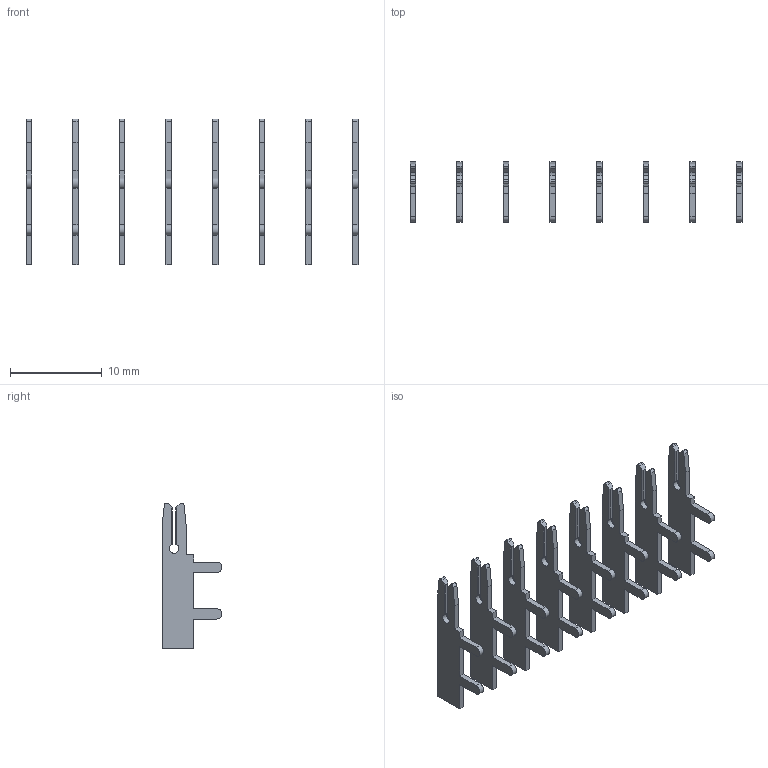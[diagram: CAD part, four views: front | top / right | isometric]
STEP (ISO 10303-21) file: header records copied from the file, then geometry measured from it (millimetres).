
FILE_DESCRIPTION (( 'STEP AP203' ), '1' );
FILE_NAME ('105-008-202-200.STEP', '2020-04-07T22:20:58', ( '' ), ( '' ), 'SwSTEP 2.0', 'SolidWorks 2016', '' );
FILE_SCHEMA (( 'CONFIG_CONTROL_DESIGN' ));
Length unit declared in the file: inch
Products named in the file (2): 100-290-001_100-290-202; 105-008-202-200
Assembly tree (8 placements, depth 2):
  105-008-202-200
    100-290-001_100-290-202  x8
Bounding box: 36.16 x 6.53 x 15.88 mm (x, y, z)
Volume: 254.2 mm3; surface area: 1130.4 mm2
Topology: 8 solids, 8 shells, 240 faces, 672 edges, 448 vertices
Faces by surface type: plane 184, cylinder 56
Entity records: 1386 total; most frequent: CARTESIAN_POINT 193, DIRECTION 176, ORIENTED_EDGE 168, EDGE_CURVE 84, LINE 66, VECTOR 66, VERTEX_POINT 56, AXIS2_PLACEMENT_3D 55
